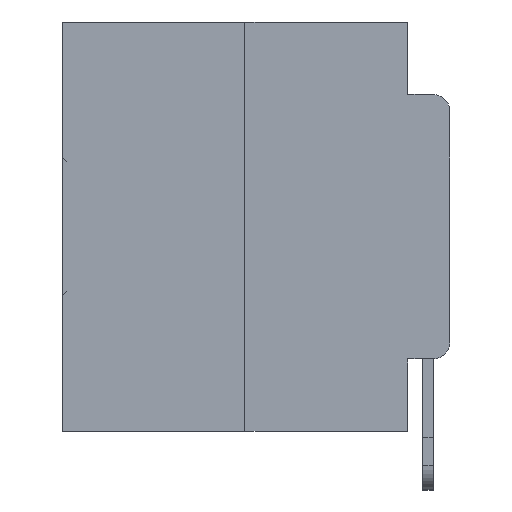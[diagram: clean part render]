
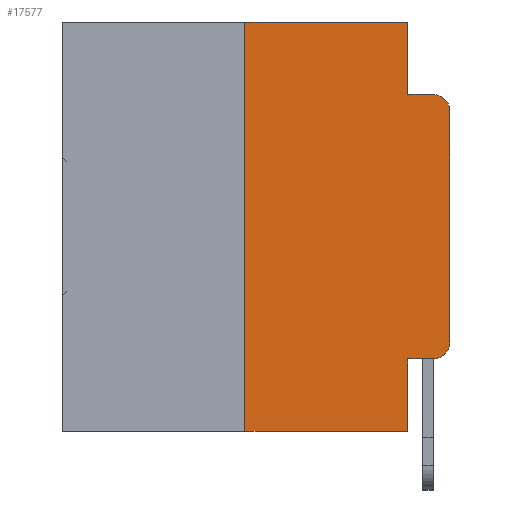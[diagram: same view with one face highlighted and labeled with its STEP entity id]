
A CAD part, left-side view. The second image highlights one B-rep face of the part: STEP entity #17577.
In plain terms, the highlighted planar face has unit normal (-1, 0, 0).
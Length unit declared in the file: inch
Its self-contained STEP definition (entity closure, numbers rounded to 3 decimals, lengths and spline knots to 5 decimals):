
#27 = VERTEX_POINT ( 'NONE', #17655 ) ;
#410 = LINE ( 'NONE', #2360, #13382 ) ;
#901 = CARTESIAN_POINT ( 'NONE',  ( 0., 0.051, -0.5 ) ) ;
#1591 = VECTOR ( 'NONE', #20281, 39.37008 ) ;
#1676 = VECTOR ( 'NONE', #9123, 39.37008 ) ;
#2360 = CARTESIAN_POINT ( 'NONE',  ( 0., 0.473, 0. ) ) ;
#2396 = LINE ( 'NONE', #2624, #1591 ) ;
#2479 = LINE ( 'NONE', #6495, #1676 ) ;
#2592 = VERTEX_POINT ( 'NONE', #901 ) ;
#2624 = CARTESIAN_POINT ( 'NONE',  ( 0., 0.473, -0.5 ) ) ;
#2847 = ORIENTED_EDGE ( 'NONE', *, *, #8487, .F. ) ;
#3628 = FACE_OUTER_BOUND ( 'NONE', #26815, .T. ) ;
#3682 = DIRECTION ( 'NONE',  ( 0., 0., 1. ) ) ;
#3779 = CARTESIAN_POINT ( 'NONE',  ( 0., 0., -0.1085 ) ) ;
#4017 = DIRECTION ( 'NONE',  ( 0., 0., -1. ) ) ;
#4340 = EDGE_CURVE ( 'NONE', #13310, #19057, #2479, .T. ) ;
#4517 = ORIENTED_EDGE ( 'NONE', *, *, #31991, .T. ) ;
#5202 = VECTOR ( 'NONE', #22686, 39.37008 ) ;
#5276 = ORIENTED_EDGE ( 'NONE', *, *, #7196, .T. ) ;
#6377 = LINE ( 'NONE', #27631, #18910 ) ;
#6394 = LINE ( 'NONE', #18335, #18928 ) ;
#6495 = CARTESIAN_POINT ( 'NONE',  ( 0., 0.051, 0. ) ) ;
#7196 = EDGE_CURVE ( 'NONE', #9797, #9636, #26475, .T. ) ;
#7400 = EDGE_CURVE ( 'NONE', #27036, #9797, #31016, .T. ) ;
#7904 = CARTESIAN_POINT ( 'NONE',  ( 0., 0.051, -0.4115 ) ) ;
#8270 = DIRECTION ( 'NONE',  ( -1., 0., 0. ) ) ;
#8487 = EDGE_CURVE ( 'NONE', #23307, #2592, #29792, .T. ) ;
#9123 = DIRECTION ( 'NONE',  ( 0., 0., -1. ) ) ;
#9621 = CARTESIAN_POINT ( 'NONE',  ( 0., 0.051, 0. ) ) ;
#9636 = VERTEX_POINT ( 'NONE', #3779 ) ;
#9797 = VERTEX_POINT ( 'NONE', #17169 ) ;
#10716 = CARTESIAN_POINT ( 'NONE',  ( 0., 0.051, 0. ) ) ;
#10970 = ORIENTED_EDGE ( 'NONE', *, *, #4340, .F. ) ;
#11173 = VECTOR ( 'NONE', #12151, 39.37008 ) ;
#11579 = CARTESIAN_POINT ( 'NONE',  ( 0., 0.25, -0.5 ) ) ;
#12151 = DIRECTION ( 'NONE',  ( 0., 0., -1. ) ) ;
#12331 = DIRECTION ( 'NONE',  ( -1., 0., 0. ) ) ;
#13225 = EDGE_CURVE ( 'NONE', #14754, #2592, #2396, .T. ) ;
#13310 = VERTEX_POINT ( 'NONE', #10716 ) ;
#13337 = ORIENTED_EDGE ( 'NONE', *, *, #31418, .F. ) ;
#13382 = VECTOR ( 'NONE', #17604, 39.37008 ) ;
#14754 = VERTEX_POINT ( 'NONE', #11579 ) ;
#15093 = AXIS2_PLACEMENT_3D ( 'NONE', #23041, #8270, #25435 ) ;
#15828 = CARTESIAN_POINT ( 'NONE',  ( 0., 0.25, 0. ) ) ;
#17169 = CARTESIAN_POINT ( 'NONE',  ( 0., 0., -0.3915 ) ) ;
#17345 = VERTEX_POINT ( 'NONE', #15828 ) ;
#17542 = ORIENTED_EDGE ( 'NONE', *, *, #29487, .F. ) ;
#17577 = ADVANCED_FACE ( 'NONE', ( #3628 ), #28657, .F. ) ;
#17604 = DIRECTION ( 'NONE',  ( 0., -1., 0. ) ) ;
#17655 = CARTESIAN_POINT ( 'NONE',  ( 0., 0.02, -0.0885 ) ) ;
#18062 = DIRECTION ( 'NONE',  ( 0., -1., 0. ) ) ;
#18335 = CARTESIAN_POINT ( 'NONE',  ( 0., 0.051, -0.4115 ) ) ;
#18910 = VECTOR ( 'NONE', #18062, 39.37008 ) ;
#18928 = VECTOR ( 'NONE', #20761, 39.37008 ) ;
#19057 = VERTEX_POINT ( 'NONE', #30940 ) ;
#19094 = DIRECTION ( 'NONE',  ( 1., 0., 0. ) ) ;
#19505 = EDGE_CURVE ( 'NONE', #19057, #27, #6377, .T. ) ;
#20169 = ORIENTED_EDGE ( 'NONE', *, *, #30816, .T. ) ;
#20255 = CARTESIAN_POINT ( 'NONE',  ( 0., 0.25, 0. ) ) ;
#20281 = DIRECTION ( 'NONE',  ( 0., -1., 0. ) ) ;
#20761 = DIRECTION ( 'NONE',  ( 0., -1., 0. ) ) ;
#21354 = ORIENTED_EDGE ( 'NONE', *, *, #13225, .T. ) ;
#21757 = AXIS2_PLACEMENT_3D ( 'NONE', #26846, #12331, #29303 ) ;
#22686 = DIRECTION ( 'NONE',  ( 0., 0., 1. ) ) ;
#23041 = CARTESIAN_POINT ( 'NONE',  ( 0., 0.02, -0.1085 ) ) ;
#23307 = VERTEX_POINT ( 'NONE', #7904 ) ;
#24081 = CARTESIAN_POINT ( 'NONE',  ( 0., 0.02, -0.4115 ) ) ;
#24357 = ORIENTED_EDGE ( 'NONE', *, *, #7400, .T. ) ;
#24980 = VECTOR ( 'NONE', #3682, 39.37008 ) ;
#24986 = LINE ( 'NONE', #20255, #5202 ) ;
#25435 = DIRECTION ( 'NONE',  ( 0., 0., -1. ) ) ;
#26475 = LINE ( 'NONE', #30803, #24980 ) ;
#26815 = EDGE_LOOP ( 'NONE', ( #5276, #20169, #28090, #10970, #17542, #13337, #21354, #2847, #4517, #24357 ) ) ;
#26846 = CARTESIAN_POINT ( 'NONE',  ( 0., 0.02, -0.3915 ) ) ;
#27036 = VERTEX_POINT ( 'NONE', #24081 ) ;
#27631 = CARTESIAN_POINT ( 'NONE',  ( 0., 0.051, -0.0885 ) ) ;
#27763 = AXIS2_PLACEMENT_3D ( 'NONE', #31102, #19094, #4017 ) ;
#28041 = CIRCLE ( 'NONE', #15093, 0.02 ) ;
#28090 = ORIENTED_EDGE ( 'NONE', *, *, #19505, .F. ) ;
#28657 = PLANE ( 'NONE',  #27763 ) ;
#29303 = DIRECTION ( 'NONE',  ( 0., 0., -1. ) ) ;
#29487 = EDGE_CURVE ( 'NONE', #17345, #13310, #410, .T. ) ;
#29792 = LINE ( 'NONE', #9621, #11173 ) ;
#30803 = CARTESIAN_POINT ( 'NONE',  ( 0., 0., 0. ) ) ;
#30816 = EDGE_CURVE ( 'NONE', #9636, #27, #28041, .T. ) ;
#30940 = CARTESIAN_POINT ( 'NONE',  ( 0., 0.051, -0.0885 ) ) ;
#31016 = CIRCLE ( 'NONE', #21757, 0.02 ) ;
#31102 = CARTESIAN_POINT ( 'NONE',  ( 0., 0.473, 0. ) ) ;
#31418 = EDGE_CURVE ( 'NONE', #14754, #17345, #24986, .T. ) ;
#31991 = EDGE_CURVE ( 'NONE', #23307, #27036, #6394, .T. ) ;
